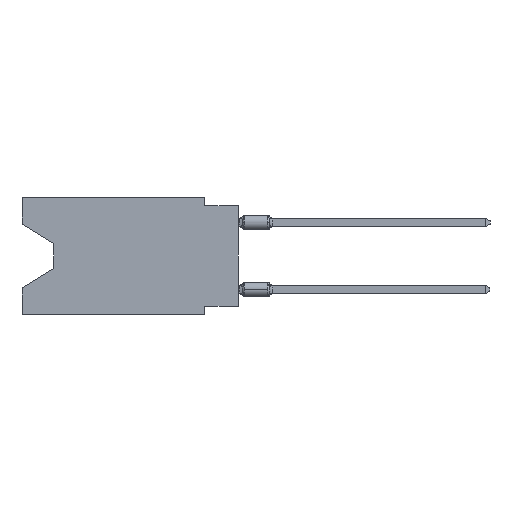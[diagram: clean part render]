
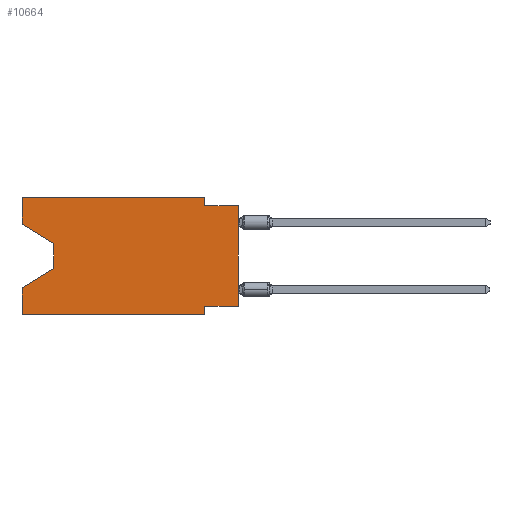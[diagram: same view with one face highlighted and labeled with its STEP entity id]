
A CAD part, left-side view. The second image highlights one B-rep face of the part: STEP entity #10664.
In plain terms, the highlighted planar face has unit normal (-1, 0, 0).
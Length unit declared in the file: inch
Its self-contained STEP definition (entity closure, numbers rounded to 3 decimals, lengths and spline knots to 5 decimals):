
#110 = CARTESIAN_POINT ( 'NONE',  ( 0., 0.645, -0.35 ) ) ;
#250 = CARTESIAN_POINT ( 'NONE',  ( 0., 0.645, -0.35 ) ) ;
#324 = VECTOR ( 'NONE', #14270, 39.37008 ) ;
#1151 = EDGE_CURVE ( 'NONE', #11257, #10757, #9709, .T. ) ;
#1517 = ORIENTED_EDGE ( 'NONE', *, *, #3224, .F. ) ;
#2110 = EDGE_CURVE ( 'NONE', #15808, #4539, #4980, .T. ) ;
#2345 = ORIENTED_EDGE ( 'NONE', *, *, #13749, .F. ) ;
#2846 = DIRECTION ( 'NONE',  ( 0., 0., -1. ) ) ;
#3029 = CARTESIAN_POINT ( 'NONE',  ( 0., 0.645, -0.08025 ) ) ;
#3224 = EDGE_CURVE ( 'NONE', #10757, #10967, #15287, .T. ) ;
#4068 = ORIENTED_EDGE ( 'NONE', *, *, #2110, .T. ) ;
#4136 = DIRECTION ( 'NONE',  ( 0., -1., 0. ) ) ;
#4174 = CARTESIAN_POINT ( 'NONE',  ( 0., 0.1, 0. ) ) ;
#4460 = EDGE_CURVE ( 'NONE', #12261, #16207, #5260, .T. ) ;
#4539 = VERTEX_POINT ( 'NONE', #8199 ) ;
#4614 = CARTESIAN_POINT ( 'NONE',  ( 0., 0.645, -0.26975 ) ) ;
#4980 = LINE ( 'NONE', #250, #15762 ) ;
#5213 = CARTESIAN_POINT ( 'NONE',  ( 0., 0.1, -0.025 ) ) ;
#5260 = LINE ( 'NONE', #8305, #15669 ) ;
#5527 = VECTOR ( 'NONE', #16908, 39.37008 ) ;
#5587 = LINE ( 'NONE', #19347, #12564 ) ;
#5784 = DIRECTION ( 'NONE',  ( 0., 0., 1. ) ) ;
#5815 = CARTESIAN_POINT ( 'NONE',  ( 0., 0.645, 0. ) ) ;
#5978 = CARTESIAN_POINT ( 'NONE',  ( 0., 0.55, -0.138 ) ) ;
#6039 = CARTESIAN_POINT ( 'NONE',  ( 0., 0.1, 0. ) ) ;
#6361 = PLANE ( 'NONE',  #19844 ) ;
#6389 = DIRECTION ( 'NONE',  ( 0., 0., 1. ) ) ;
#6400 = DIRECTION ( 'NONE',  ( 0., -1., 0. ) ) ;
#6541 = VERTEX_POINT ( 'NONE', #7379 ) ;
#6875 = VECTOR ( 'NONE', #15601, 39.37008 ) ;
#7167 = EDGE_CURVE ( 'NONE', #18257, #12036, #10940, .T. ) ;
#7379 = CARTESIAN_POINT ( 'NONE',  ( 0., 0.1, -0.325 ) ) ;
#7759 = FACE_OUTER_BOUND ( 'NONE', #18010, .T. ) ;
#8009 = DIRECTION ( 'NONE',  ( 0., 0.855, -0.519 ) ) ;
#8084 = CARTESIAN_POINT ( 'NONE',  ( 0., 0.55, -0.138 ) ) ;
#8199 = CARTESIAN_POINT ( 'NONE',  ( 0., 0.1, -0.35 ) ) ;
#8240 = ORIENTED_EDGE ( 'NONE', *, *, #17796, .T. ) ;
#8305 = CARTESIAN_POINT ( 'NONE',  ( 0., 0.55, -0.212 ) ) ;
#9573 = ORIENTED_EDGE ( 'NONE', *, *, #13866, .F. ) ;
#9709 = LINE ( 'NONE', #14172, #324 ) ;
#9862 = VECTOR ( 'NONE', #2846, 39.37008 ) ;
#9916 = CARTESIAN_POINT ( 'NONE',  ( 0., 0., -0.025 ) ) ;
#10293 = CARTESIAN_POINT ( 'NONE',  ( 0., 0., -0.025 ) ) ;
#10372 = VERTEX_POINT ( 'NONE', #3029 ) ;
#10621 = VECTOR ( 'NONE', #17139, 39.37008 ) ;
#10664 = ADVANCED_FACE ( 'NONE', ( #7759 ), #6361, .F. ) ;
#10669 = ORIENTED_EDGE ( 'NONE', *, *, #12789, .F. ) ;
#10757 = VERTEX_POINT ( 'NONE', #6039 ) ;
#10940 = LINE ( 'NONE', #14069, #15647 ) ;
#10967 = VERTEX_POINT ( 'NONE', #5213 ) ;
#11170 = LINE ( 'NONE', #14400, #10621 ) ;
#11257 = VERTEX_POINT ( 'NONE', #16921 ) ;
#11327 = ORIENTED_EDGE ( 'NONE', *, *, #19163, .T. ) ;
#11492 = EDGE_CURVE ( 'NONE', #6541, #4539, #11170, .T. ) ;
#11745 = DIRECTION ( 'NONE',  ( 0., 1., 0. ) ) ;
#11948 = LINE ( 'NONE', #19644, #12871 ) ;
#11949 = ORIENTED_EDGE ( 'NONE', *, *, #7167, .T. ) ;
#12011 = CARTESIAN_POINT ( 'NONE',  ( 0., 0., -0.325 ) ) ;
#12036 = VERTEX_POINT ( 'NONE', #9916 ) ;
#12199 = DIRECTION ( 'NONE',  ( 1., 0., 0. ) ) ;
#12261 = VERTEX_POINT ( 'NONE', #15661 ) ;
#12564 = VECTOR ( 'NONE', #11745, 39.37008 ) ;
#12789 = EDGE_CURVE ( 'NONE', #10967, #12036, #16668, .T. ) ;
#12871 = VECTOR ( 'NONE', #5784, 39.37008 ) ;
#13187 = VECTOR ( 'NONE', #18460, 39.37008 ) ;
#13339 = ORIENTED_EDGE ( 'NONE', *, *, #1151, .F. ) ;
#13508 = LINE ( 'NONE', #5815, #13187 ) ;
#13749 = EDGE_CURVE ( 'NONE', #18257, #6541, #5587, .T. ) ;
#13819 = DIRECTION ( 'NONE',  ( 0., 0., -1. ) ) ;
#13866 = EDGE_CURVE ( 'NONE', #15808, #16207, #11948, .T. ) ;
#14069 = CARTESIAN_POINT ( 'NONE',  ( 0., 0., 0. ) ) ;
#14172 = CARTESIAN_POINT ( 'NONE',  ( 0., 0.645, 0. ) ) ;
#14270 = DIRECTION ( 'NONE',  ( 0., -1., 0. ) ) ;
#14400 = CARTESIAN_POINT ( 'NONE',  ( 0., 0.1, -0.35 ) ) ;
#14594 = EDGE_CURVE ( 'NONE', #10372, #11257, #13508, .T. ) ;
#15146 = CARTESIAN_POINT ( 'NONE',  ( 0., 0.645, 0. ) ) ;
#15287 = LINE ( 'NONE', #4174, #5527 ) ;
#15421 = VECTOR ( 'NONE', #4136, 39.37008 ) ;
#15601 = DIRECTION ( 'NONE',  ( 0., -0.855, -0.519 ) ) ;
#15647 = VECTOR ( 'NONE', #6389, 39.37008 ) ;
#15661 = CARTESIAN_POINT ( 'NONE',  ( 0., 0.55, -0.212 ) ) ;
#15669 = VECTOR ( 'NONE', #8009, 39.37008 ) ;
#15762 = VECTOR ( 'NONE', #6400, 39.37008 ) ;
#15808 = VERTEX_POINT ( 'NONE', #110 ) ;
#15818 = ORIENTED_EDGE ( 'NONE', *, *, #14594, .F. ) ;
#16207 = VERTEX_POINT ( 'NONE', #4614 ) ;
#16592 = LINE ( 'NONE', #5978, #9862 ) ;
#16665 = VERTEX_POINT ( 'NONE', #8084 ) ;
#16668 = LINE ( 'NONE', #10293, #15421 ) ;
#16908 = DIRECTION ( 'NONE',  ( 0., 0., -1. ) ) ;
#16921 = CARTESIAN_POINT ( 'NONE',  ( 0., 0.645, 0. ) ) ;
#17138 = ORIENTED_EDGE ( 'NONE', *, *, #11492, .F. ) ;
#17139 = DIRECTION ( 'NONE',  ( 0., 0., -1. ) ) ;
#17796 = EDGE_CURVE ( 'NONE', #16665, #12261, #16592, .T. ) ;
#18010 = EDGE_LOOP ( 'NONE', ( #11327, #8240, #18793, #9573, #4068, #17138, #2345, #11949, #10669, #1517, #13339, #15818 ) ) ;
#18257 = VERTEX_POINT ( 'NONE', #12011 ) ;
#18460 = DIRECTION ( 'NONE',  ( 0., 0., 1. ) ) ;
#18528 = CARTESIAN_POINT ( 'NONE',  ( 0., 0.645, -0.08025 ) ) ;
#18793 = ORIENTED_EDGE ( 'NONE', *, *, #4460, .T. ) ;
#19163 = EDGE_CURVE ( 'NONE', #10372, #16665, #19959, .T. ) ;
#19347 = CARTESIAN_POINT ( 'NONE',  ( 0., 0., -0.325 ) ) ;
#19644 = CARTESIAN_POINT ( 'NONE',  ( 0., 0.645, 0. ) ) ;
#19844 = AXIS2_PLACEMENT_3D ( 'NONE', #15146, #12199, #13819 ) ;
#19959 = LINE ( 'NONE', #18528, #6875 ) ;
